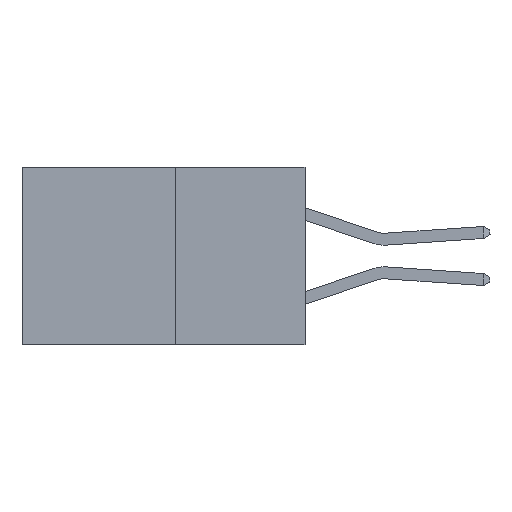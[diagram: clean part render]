
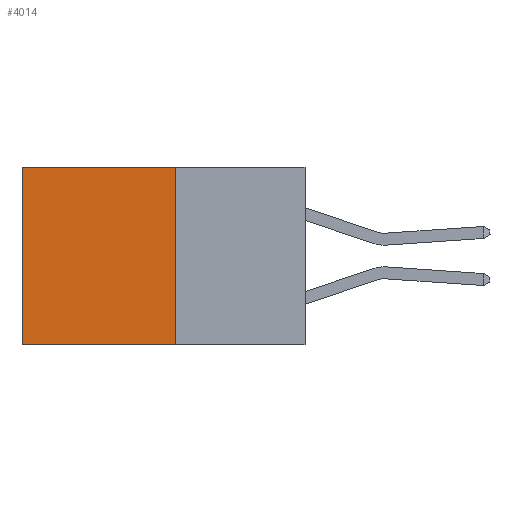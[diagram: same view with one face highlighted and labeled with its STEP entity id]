
A CAD part, left-side view. The second image highlights one B-rep face of the part: STEP entity #4014.
In plain terms, the highlighted planar face has unit normal (-1, 0, 0).
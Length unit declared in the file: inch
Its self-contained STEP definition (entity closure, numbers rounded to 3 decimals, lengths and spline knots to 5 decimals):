
#913 = VERTEX_POINT ( 'NONE', #15061 ) ;
#1675 = EDGE_CURVE ( 'NONE', #18495, #2186, #15734, .T. ) ;
#1977 = ORIENTED_EDGE ( 'NONE', *, *, #1675, .T. ) ;
#2186 = VERTEX_POINT ( 'NONE', #5412 ) ;
#2657 = ORIENTED_EDGE ( 'NONE', *, *, #8066, .F. ) ;
#2674 = CARTESIAN_POINT ( 'NONE',  ( 0.277, 0.27, -0.37 ) ) ;
#4014 = ADVANCED_FACE ( 'NONE', ( #13485 ), #6284, .F. ) ;
#4056 = DIRECTION ( 'NONE',  ( 0., 1., 0. ) ) ;
#4078 = EDGE_CURVE ( 'NONE', #913, #2186, #8552, .T. ) ;
#4221 = VERTEX_POINT ( 'NONE', #13364 ) ;
#4402 = VECTOR ( 'NONE', #16819, 39.37008 ) ;
#4670 = EDGE_LOOP ( 'NONE', ( #1977, #11637, #2657, #19372 ) ) ;
#4847 = CARTESIAN_POINT ( 'NONE',  ( 0.277, 0.59, 0. ) ) ;
#5412 = CARTESIAN_POINT ( 'NONE',  ( 0.277, 0.59, -0.37 ) ) ;
#6284 = PLANE ( 'NONE',  #11714 ) ;
#6890 = EDGE_CURVE ( 'NONE', #4221, #18495, #12555, .T. ) ;
#7098 = LINE ( 'NONE', #11212, #14654 ) ;
#8066 = EDGE_CURVE ( 'NONE', #4221, #913, #7098, .T. ) ;
#8552 = LINE ( 'NONE', #10923, #12086 ) ;
#10271 = DIRECTION ( 'NONE',  ( 0., 0., -1. ) ) ;
#10923 = CARTESIAN_POINT ( 'NONE',  ( 0.277, 0.27, -0.37 ) ) ;
#11151 = DIRECTION ( 'NONE',  ( 0., 0., -1. ) ) ;
#11212 = CARTESIAN_POINT ( 'NONE',  ( 0.277, 0.27, -0.37 ) ) ;
#11637 = ORIENTED_EDGE ( 'NONE', *, *, #4078, .F. ) ;
#11714 = AXIS2_PLACEMENT_3D ( 'NONE', #2674, #19199, #18896 ) ;
#11746 = VECTOR ( 'NONE', #10271, 39.37008 ) ;
#12086 = VECTOR ( 'NONE', #4056, 39.37008 ) ;
#12555 = LINE ( 'NONE', #19294, #4402 ) ;
#13364 = CARTESIAN_POINT ( 'NONE',  ( 0.277, 0.27, 0. ) ) ;
#13485 = FACE_OUTER_BOUND ( 'NONE', #4670, .T. ) ;
#14654 = VECTOR ( 'NONE', #11151, 39.37008 ) ;
#15061 = CARTESIAN_POINT ( 'NONE',  ( 0.277, 0.27, -0.37 ) ) ;
#15734 = LINE ( 'NONE', #19039, #11746 ) ;
#16819 = DIRECTION ( 'NONE',  ( 0., 1., 0. ) ) ;
#18495 = VERTEX_POINT ( 'NONE', #4847 ) ;
#18896 = DIRECTION ( 'NONE',  ( 0., 0., -1. ) ) ;
#19039 = CARTESIAN_POINT ( 'NONE',  ( 0.277, 0.59, -0.37 ) ) ;
#19199 = DIRECTION ( 'NONE',  ( 1., 0., 0. ) ) ;
#19294 = CARTESIAN_POINT ( 'NONE',  ( 0.277, 0.27, 0. ) ) ;
#19372 = ORIENTED_EDGE ( 'NONE', *, *, #6890, .T. ) ;
